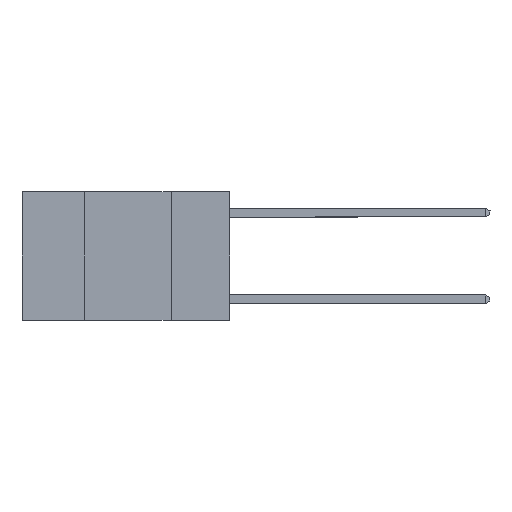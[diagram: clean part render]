
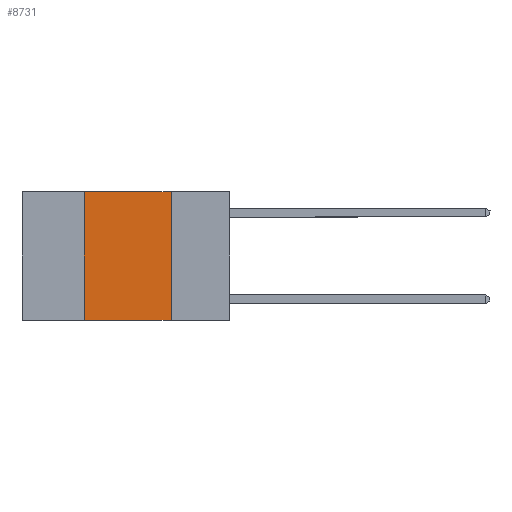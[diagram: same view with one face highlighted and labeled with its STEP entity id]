
A CAD part, left-side view. The second image highlights one B-rep face of the part: STEP entity #8731.
In plain terms, the highlighted planar face has unit normal (-1, 0, 0).
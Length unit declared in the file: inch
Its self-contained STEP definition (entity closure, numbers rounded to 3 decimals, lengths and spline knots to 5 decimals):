
#653 = DIRECTION ( 'NONE',  ( 1., 0., 0. ) ) ;
#1572 = CARTESIAN_POINT ( 'NONE',  ( 0., 0.17, 0. ) ) ;
#1679 = DIRECTION ( 'NONE',  ( 0., -1., 0. ) ) ;
#1817 = CARTESIAN_POINT ( 'NONE',  ( 0., 0.17, -0.37 ) ) ;
#2427 = CARTESIAN_POINT ( 'NONE',  ( 0., 0.6, 0. ) ) ;
#2499 = VERTEX_POINT ( 'NONE', #5050 ) ;
#2767 = ORIENTED_EDGE ( 'NONE', *, *, #8783, .F. ) ;
#2972 = VERTEX_POINT ( 'NONE', #1817 ) ;
#3306 = VERTEX_POINT ( 'NONE', #7992 ) ;
#3607 = VECTOR ( 'NONE', #1679, 39.37008 ) ;
#3706 = VECTOR ( 'NONE', #6410, 39.37008 ) ;
#4133 = CARTESIAN_POINT ( 'NONE',  ( 0., 0.6, -0.37 ) ) ;
#4417 = CARTESIAN_POINT ( 'NONE',  ( 0., 0.42, -0.37 ) ) ;
#4462 = FACE_OUTER_BOUND ( 'NONE', #9591, .T. ) ;
#4550 = ORIENTED_EDGE ( 'NONE', *, *, #5985, .F. ) ;
#5050 = CARTESIAN_POINT ( 'NONE',  ( 0., 0.17, 0. ) ) ;
#5491 = ORIENTED_EDGE ( 'NONE', *, *, #7676, .T. ) ;
#5559 = LINE ( 'NONE', #2427, #3706 ) ;
#5709 = LINE ( 'NONE', #4133, #3607 ) ;
#5985 = EDGE_CURVE ( 'NONE', #9033, #3306, #7799, .T. ) ;
#6056 = VECTOR ( 'NONE', #6377, 39.37008 ) ;
#6377 = DIRECTION ( 'NONE',  ( 0., 0., -1. ) ) ;
#6410 = DIRECTION ( 'NONE',  ( 0., -1., 0. ) ) ;
#6877 = DIRECTION ( 'NONE',  ( 0., 0., 1. ) ) ;
#7676 = EDGE_CURVE ( 'NONE', #9033, #2972, #5709, .T. ) ;
#7799 = LINE ( 'NONE', #8511, #9718 ) ;
#7910 = CARTESIAN_POINT ( 'NONE',  ( 0., 0.6, 0. ) ) ;
#7992 = CARTESIAN_POINT ( 'NONE',  ( 0., 0.42, 0. ) ) ;
#8367 = EDGE_CURVE ( 'NONE', #2499, #2972, #10393, .T. ) ;
#8511 = CARTESIAN_POINT ( 'NONE',  ( 0., 0.42, 0. ) ) ;
#8731 = ADVANCED_FACE ( 'NONE', ( #4462 ), #8737, .F. ) ;
#8737 = PLANE ( 'NONE',  #9541 ) ;
#8783 = EDGE_CURVE ( 'NONE', #3306, #2499, #5559, .T. ) ;
#9033 = VERTEX_POINT ( 'NONE', #4417 ) ;
#9541 = AXIS2_PLACEMENT_3D ( 'NONE', #7910, #653, #9552 ) ;
#9552 = DIRECTION ( 'NONE',  ( 0., 0., -1. ) ) ;
#9591 = EDGE_LOOP ( 'NONE', ( #10272, #2767, #4550, #5491 ) ) ;
#9718 = VECTOR ( 'NONE', #6877, 39.37008 ) ;
#10272 = ORIENTED_EDGE ( 'NONE', *, *, #8367, .F. ) ;
#10393 = LINE ( 'NONE', #1572, #6056 ) ;
